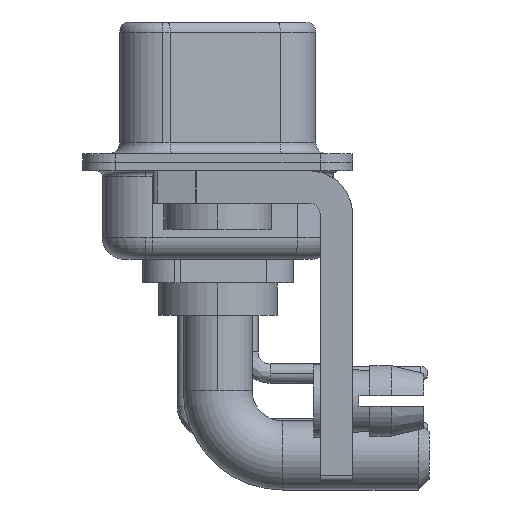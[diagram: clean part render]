
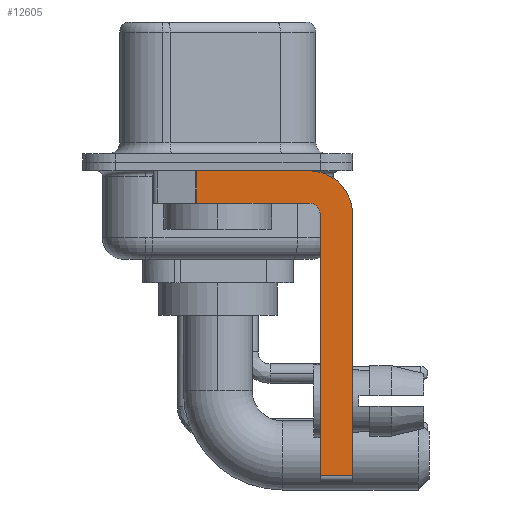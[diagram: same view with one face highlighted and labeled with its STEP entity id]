
A CAD part, left-side view. The second image highlights one B-rep face of the part: STEP entity #12605.
In plain terms, the highlighted planar face has unit normal (-1, 0, 0).
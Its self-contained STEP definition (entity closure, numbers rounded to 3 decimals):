
#185 = DIRECTION ( 'NONE',  ( 0., 0., -1. ) ) ;
#487 = VERTEX_POINT ( 'NONE', #24854 ) ;
#601 = DIRECTION ( 'NONE',  ( 0., 0., 1. ) ) ;
#944 = EDGE_CURVE ( 'NONE', #11870, #487, #3538, .T. ) ;
#1957 = DIRECTION ( 'NONE',  ( 1., 0., 0. ) ) ;
#2289 = DIRECTION ( 'NONE',  ( 0., -1., 0. ) ) ;
#2381 = VERTEX_POINT ( 'NONE', #9527 ) ;
#3078 = VECTOR ( 'NONE', #14151, 1000. ) ;
#3186 = VERTEX_POINT ( 'NONE', #19689 ) ;
#3538 = LINE ( 'NONE', #10494, #8363 ) ;
#4038 = EDGE_LOOP ( 'NONE', ( #11892, #16258, #18432, #13895, #11441, #6706, #20283, #16504 ) ) ;
#4356 = DIRECTION ( 'NONE',  ( 0., 0., -1. ) ) ;
#4818 = DIRECTION ( 'NONE',  ( 0., 1., 0. ) ) ;
#5634 = CARTESIAN_POINT ( 'NONE',  ( -2.9, 3., -0.4 ) ) ;
#6050 = DIRECTION ( 'NONE',  ( 0., 0., -1. ) ) ;
#6706 = ORIENTED_EDGE ( 'NONE', *, *, #944, .T. ) ;
#7834 = EDGE_CURVE ( 'NONE', #25080, #2381, #10118, .T. ) ;
#8042 = CARTESIAN_POINT ( 'NONE',  ( -2.9, -4.25, -0.4 ) ) ;
#8363 = VECTOR ( 'NONE', #2289, 1000. ) ;
#8462 = DIRECTION ( 'NONE',  ( 1., 0., 0. ) ) ;
#8545 = VECTOR ( 'NONE', #21471, 1000. ) ;
#9060 = EDGE_CURVE ( 'NONE', #25080, #16440, #11987, .T. ) ;
#9175 = LINE ( 'NONE', #17239, #8545 ) ;
#9370 = EDGE_CURVE ( 'NONE', #19841, #2381, #19110, .T. ) ;
#9527 = CARTESIAN_POINT ( 'NONE',  ( -2.9, 0.978, -1.9 ) ) ;
#9544 = VECTOR ( 'NONE', #24020, 1000. ) ;
#9789 = CARTESIAN_POINT ( 'NONE',  ( -2.9, 0.978, -0.4 ) ) ;
#10118 = LINE ( 'NONE', #20181, #12877 ) ;
#10166 = LINE ( 'NONE', #20352, #3078 ) ;
#10494 = CARTESIAN_POINT ( 'NONE',  ( -2.9, -4.25, -14.55 ) ) ;
#11161 = CARTESIAN_POINT ( 'NONE',  ( -2.9, -4.25, -1.9 ) ) ;
#11181 = CARTESIAN_POINT ( 'NONE',  ( -2.9, -4.25, -1.9 ) ) ;
#11441 = ORIENTED_EDGE ( 'NONE', *, *, #19845, .F. ) ;
#11690 = AXIS2_PLACEMENT_3D ( 'NONE', #26169, #1957, #6050 ) ;
#11870 = VERTEX_POINT ( 'NONE', #20870 ) ;
#11892 = ORIENTED_EDGE ( 'NONE', *, *, #9060, .F. ) ;
#11987 = LINE ( 'NONE', #5634, #9544 ) ;
#12605 = ADVANCED_FACE ( 'NONE', ( #22354 ), #22481, .F. ) ;
#12877 = VECTOR ( 'NONE', #185, 1000. ) ;
#13730 = CIRCLE ( 'NONE', #17088, 0.5 ) ;
#13895 = ORIENTED_EDGE ( 'NONE', *, *, #23727, .F. ) ;
#14151 = DIRECTION ( 'NONE',  ( 0., 0., -1. ) ) ;
#16258 = ORIENTED_EDGE ( 'NONE', *, *, #7834, .T. ) ;
#16385 = AXIS2_PLACEMENT_3D ( 'NONE', #16519, #8462, #4356 ) ;
#16440 = VERTEX_POINT ( 'NONE', #8042 ) ;
#16475 = VERTEX_POINT ( 'NONE', #23925 ) ;
#16504 = ORIENTED_EDGE ( 'NONE', *, *, #25618, .F. ) ;
#16519 = CARTESIAN_POINT ( 'NONE',  ( -2.9, -4.25, -2.4 ) ) ;
#17088 = AXIS2_PLACEMENT_3D ( 'NONE', #18732, #24952, #601 ) ;
#17239 = CARTESIAN_POINT ( 'NONE',  ( -2.9, -4.75, -14.8 ) ) ;
#18432 = ORIENTED_EDGE ( 'NONE', *, *, #9370, .F. ) ;
#18732 = CARTESIAN_POINT ( 'NONE',  ( -2.9, -4.25, -2.4 ) ) ;
#19110 = LINE ( 'NONE', #11181, #20529 ) ;
#19689 = CARTESIAN_POINT ( 'NONE',  ( -2.9, -6.25, -2.4 ) ) ;
#19841 = VERTEX_POINT ( 'NONE', #11161 ) ;
#19845 = EDGE_CURVE ( 'NONE', #11870, #16475, #9175, .T. ) ;
#20181 = CARTESIAN_POINT ( 'NONE',  ( -2.9, 0.978, -1.9 ) ) ;
#20283 = ORIENTED_EDGE ( 'NONE', *, *, #20463, .F. ) ;
#20352 = CARTESIAN_POINT ( 'NONE',  ( -2.9, -6.25, -2.4 ) ) ;
#20463 = EDGE_CURVE ( 'NONE', #3186, #487, #10166, .T. ) ;
#20529 = VECTOR ( 'NONE', #4818, 1000. ) ;
#20870 = CARTESIAN_POINT ( 'NONE',  ( -2.9, -4.75, -14.55 ) ) ;
#21471 = DIRECTION ( 'NONE',  ( 0., 0., 1. ) ) ;
#22354 = FACE_OUTER_BOUND ( 'NONE', #4038, .T. ) ;
#22481 = PLANE ( 'NONE',  #16385 ) ;
#23104 = CIRCLE ( 'NONE', #11690, 2. ) ;
#23727 = EDGE_CURVE ( 'NONE', #16475, #19841, #13730, .T. ) ;
#23925 = CARTESIAN_POINT ( 'NONE',  ( -2.9, -4.75, -2.4 ) ) ;
#24020 = DIRECTION ( 'NONE',  ( 0., -1., 0. ) ) ;
#24854 = CARTESIAN_POINT ( 'NONE',  ( -2.9, -6.25, -14.55 ) ) ;
#24952 = DIRECTION ( 'NONE',  ( -1., 0., 0. ) ) ;
#25080 = VERTEX_POINT ( 'NONE', #9789 ) ;
#25618 = EDGE_CURVE ( 'NONE', #16440, #3186, #23104, .T. ) ;
#26169 = CARTESIAN_POINT ( 'NONE',  ( -2.9, -4.25, -2.4 ) ) ;
